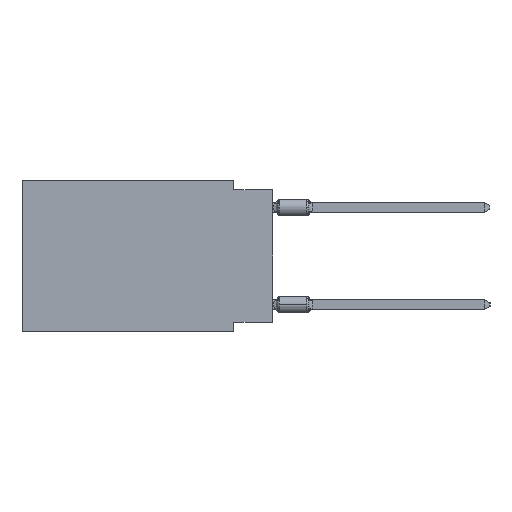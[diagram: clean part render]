
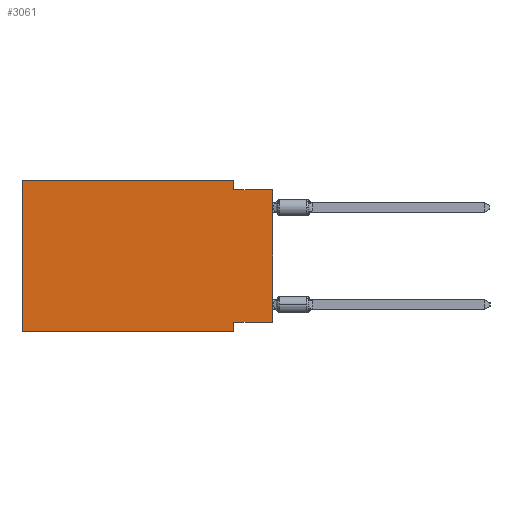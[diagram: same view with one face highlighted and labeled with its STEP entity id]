
A CAD part, left-side view. The second image highlights one B-rep face of the part: STEP entity #3061.
In plain terms, the highlighted planar face has unit normal (-1, 0, 0).
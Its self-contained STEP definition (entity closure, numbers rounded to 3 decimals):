
#914 = ORIENTED_EDGE ( 'NONE', *, *, #40065, .F. ) ;
#1586 = DIRECTION ( 'NONE',  ( 0., 0., 1. ) ) ;
#2147 = CARTESIAN_POINT ( 'NONE',  ( 0., 2.54, -9.271 ) ) ;
#3061 = ADVANCED_FACE ( 'NONE', ( #38599 ), #59245, .F. ) ;
#4904 = CARTESIAN_POINT ( 'NONE',  ( 0., 0., -0.635 ) ) ;
#5276 = VERTEX_POINT ( 'NONE', #4904 ) ;
#6861 = LINE ( 'NONE', #7177, #24957 ) ;
#6976 = VERTEX_POINT ( 'NONE', #19945 ) ;
#7177 = CARTESIAN_POINT ( 'NONE',  ( 0., 2.54, 0. ) ) ;
#8516 = CARTESIAN_POINT ( 'NONE',  ( 0., 16.383, 0. ) ) ;
#8613 = CARTESIAN_POINT ( 'NONE',  ( 0., 16.383, 0. ) ) ;
#8857 = EDGE_CURVE ( 'NONE', #6976, #31260, #52301, .T. ) ;
#9896 = EDGE_CURVE ( 'NONE', #6976, #62554, #43906, .T. ) ;
#10482 = LINE ( 'NONE', #49820, #46565 ) ;
#12433 = DIRECTION ( 'NONE',  ( 0., 0., -1. ) ) ;
#12948 = CARTESIAN_POINT ( 'NONE',  ( 0., 16.383, -9.906 ) ) ;
#13696 = DIRECTION ( 'NONE',  ( 1., 0., 0. ) ) ;
#15089 = CARTESIAN_POINT ( 'NONE',  ( 0., 0., -0.635 ) ) ;
#17388 = VERTEX_POINT ( 'NONE', #63949 ) ;
#19945 = CARTESIAN_POINT ( 'NONE',  ( 0., 16.383, -9.906 ) ) ;
#20668 = VECTOR ( 'NONE', #12433, 1000. ) ;
#20871 = VECTOR ( 'NONE', #42132, 1000. ) ;
#23185 = ORIENTED_EDGE ( 'NONE', *, *, #47041, .T. ) ;
#24957 = VECTOR ( 'NONE', #62259, 1000. ) ;
#25597 = VERTEX_POINT ( 'NONE', #32820 ) ;
#26055 = ORIENTED_EDGE ( 'NONE', *, *, #8857, .T. ) ;
#27057 = LINE ( 'NONE', #31333, #54094 ) ;
#27177 = EDGE_CURVE ( 'NONE', #47357, #31260, #42273, .T. ) ;
#28370 = AXIS2_PLACEMENT_3D ( 'NONE', #29420, #13696, #33366 ) ;
#28455 = ORIENTED_EDGE ( 'NONE', *, *, #29892, .F. ) ;
#29420 = CARTESIAN_POINT ( 'NONE',  ( 0., 16.383, 0. ) ) ;
#29892 = EDGE_CURVE ( 'NONE', #25597, #34262, #6861, .T. ) ;
#30470 = DIRECTION ( 'NONE',  ( 0., -1., 0. ) ) ;
#31260 = VERTEX_POINT ( 'NONE', #33065 ) ;
#31333 = CARTESIAN_POINT ( 'NONE',  ( 0., 0., -9.271 ) ) ;
#32706 = ORIENTED_EDGE ( 'NONE', *, *, #38916, .F. ) ;
#32820 = CARTESIAN_POINT ( 'NONE',  ( 0., 2.54, 0. ) ) ;
#33065 = CARTESIAN_POINT ( 'NONE',  ( 0., 2.54, -9.906 ) ) ;
#33366 = DIRECTION ( 'NONE',  ( 0., 0., -1. ) ) ;
#34262 = VERTEX_POINT ( 'NONE', #38864 ) ;
#35072 = DIRECTION ( 'NONE',  ( 0., -1., 0. ) ) ;
#35081 = EDGE_LOOP ( 'NONE', ( #23185, #914, #28455, #32706, #54058, #26055, #43770, #63759 ) ) ;
#35606 = VECTOR ( 'NONE', #54724, 1000. ) ;
#36213 = VECTOR ( 'NONE', #35072, 1000. ) ;
#38599 = FACE_OUTER_BOUND ( 'NONE', #35081, .T. ) ;
#38864 = CARTESIAN_POINT ( 'NONE',  ( 0., 2.54, -0.635 ) ) ;
#38916 = EDGE_CURVE ( 'NONE', #62554, #25597, #10482, .T. ) ;
#40065 = EDGE_CURVE ( 'NONE', #34262, #5276, #45569, .T. ) ;
#42132 = DIRECTION ( 'NONE',  ( 0., -1., 0. ) ) ;
#42273 = LINE ( 'NONE', #57032, #20668 ) ;
#43770 = ORIENTED_EDGE ( 'NONE', *, *, #27177, .F. ) ;
#43906 = LINE ( 'NONE', #8516, #35606 ) ;
#45569 = LINE ( 'NONE', #15089, #36213 ) ;
#46522 = LINE ( 'NONE', #56679, #63884 ) ;
#46565 = VECTOR ( 'NONE', #30470, 1000. ) ;
#47041 = EDGE_CURVE ( 'NONE', #17388, #5276, #46522, .T. ) ;
#47050 = DIRECTION ( 'NONE',  ( 0., 1., 0. ) ) ;
#47357 = VERTEX_POINT ( 'NONE', #2147 ) ;
#49820 = CARTESIAN_POINT ( 'NONE',  ( 0., 16.383, 0. ) ) ;
#52301 = LINE ( 'NONE', #12948, #20871 ) ;
#53191 = EDGE_CURVE ( 'NONE', #17388, #47357, #27057, .T. ) ;
#54058 = ORIENTED_EDGE ( 'NONE', *, *, #9896, .F. ) ;
#54094 = VECTOR ( 'NONE', #47050, 1000. ) ;
#54724 = DIRECTION ( 'NONE',  ( 0., 0., 1. ) ) ;
#56679 = CARTESIAN_POINT ( 'NONE',  ( 0., 0., 0. ) ) ;
#57032 = CARTESIAN_POINT ( 'NONE',  ( 0., 2.54, -9.906 ) ) ;
#59245 = PLANE ( 'NONE',  #28370 ) ;
#62259 = DIRECTION ( 'NONE',  ( 0., 0., -1. ) ) ;
#62554 = VERTEX_POINT ( 'NONE', #8613 ) ;
#63759 = ORIENTED_EDGE ( 'NONE', *, *, #53191, .F. ) ;
#63884 = VECTOR ( 'NONE', #1586, 1000. ) ;
#63949 = CARTESIAN_POINT ( 'NONE',  ( 0., 0., -9.271 ) ) ;
